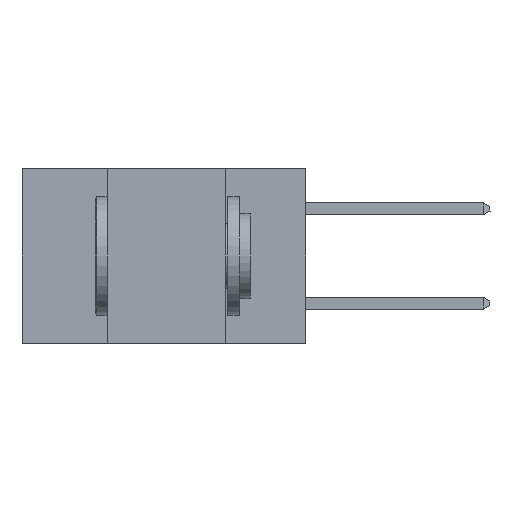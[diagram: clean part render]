
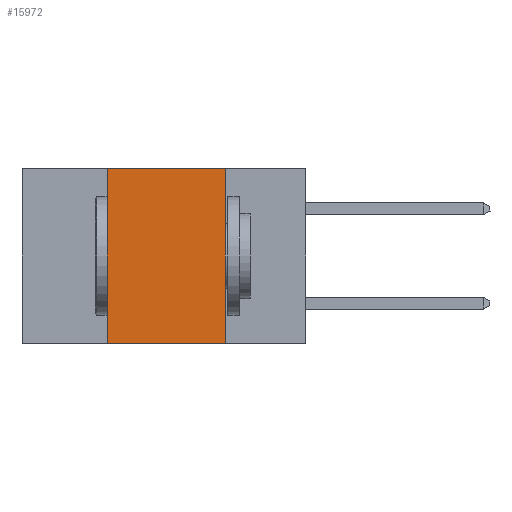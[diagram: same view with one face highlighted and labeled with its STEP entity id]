
A CAD part, left-side view. The second image highlights one B-rep face of the part: STEP entity #15972.
In plain terms, the highlighted planar face has unit normal (-1, 0, 0).
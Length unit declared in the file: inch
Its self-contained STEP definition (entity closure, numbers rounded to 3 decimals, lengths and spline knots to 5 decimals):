
#938 = DIRECTION ( 'NONE',  ( 0., 0., -1. ) ) ;
#1566 = VERTEX_POINT ( 'NONE', #9839 ) ;
#1702 = EDGE_CURVE ( 'NONE', #15841, #10804, #4116, .T. ) ;
#2092 = LINE ( 'NONE', #13589, #2477 ) ;
#2417 = ORIENTED_EDGE ( 'NONE', *, *, #7214, .T. ) ;
#2477 = VECTOR ( 'NONE', #14834, 39.37008 ) ;
#2841 = EDGE_LOOP ( 'NONE', ( #12056, #16413, #3337, #2417 ) ) ;
#3133 = CARTESIAN_POINT ( 'NONE',  ( 0., 0.42, 0. ) ) ;
#3337 = ORIENTED_EDGE ( 'NONE', *, *, #3378, .F. ) ;
#3378 = EDGE_CURVE ( 'NONE', #1566, #9306, #16498, .T. ) ;
#4116 = LINE ( 'NONE', #9894, #16558 ) ;
#4588 = DIRECTION ( 'NONE',  ( 0., -1., 0. ) ) ;
#4719 = CARTESIAN_POINT ( 'NONE',  ( 0., 0.6, 0. ) ) ;
#5078 = CARTESIAN_POINT ( 'NONE',  ( 0., 0.42, 0. ) ) ;
#7214 = EDGE_CURVE ( 'NONE', #1566, #10804, #15994, .T. ) ;
#7483 = DIRECTION ( 'NONE',  ( 0., 0., 1. ) ) ;
#7895 = FACE_OUTER_BOUND ( 'NONE', #2841, .T. ) ;
#8404 = CARTESIAN_POINT ( 'NONE',  ( 0., 0.6, -0.37 ) ) ;
#9306 = VERTEX_POINT ( 'NONE', #3133 ) ;
#9507 = PLANE ( 'NONE',  #12955 ) ;
#9690 = EDGE_CURVE ( 'NONE', #9306, #15841, #2092, .T. ) ;
#9839 = CARTESIAN_POINT ( 'NONE',  ( 0., 0.42, -0.37 ) ) ;
#9894 = CARTESIAN_POINT ( 'NONE',  ( 0., 0.17, 0. ) ) ;
#10804 = VERTEX_POINT ( 'NONE', #12071 ) ;
#11000 = CARTESIAN_POINT ( 'NONE',  ( 0., 0.17, 0. ) ) ;
#12056 = ORIENTED_EDGE ( 'NONE', *, *, #1702, .F. ) ;
#12071 = CARTESIAN_POINT ( 'NONE',  ( 0., 0.17, -0.37 ) ) ;
#12361 = VECTOR ( 'NONE', #4588, 39.37008 ) ;
#12955 = AXIS2_PLACEMENT_3D ( 'NONE', #4719, #13684, #938 ) ;
#13589 = CARTESIAN_POINT ( 'NONE',  ( 0., 0.6, 0. ) ) ;
#13684 = DIRECTION ( 'NONE',  ( 1., 0., 0. ) ) ;
#13706 = DIRECTION ( 'NONE',  ( 0., 0., -1. ) ) ;
#14692 = VECTOR ( 'NONE', #7483, 39.37008 ) ;
#14834 = DIRECTION ( 'NONE',  ( 0., -1., 0. ) ) ;
#15841 = VERTEX_POINT ( 'NONE', #11000 ) ;
#15972 = ADVANCED_FACE ( 'NONE', ( #7895 ), #9507, .F. ) ;
#15994 = LINE ( 'NONE', #8404, #12361 ) ;
#16413 = ORIENTED_EDGE ( 'NONE', *, *, #9690, .F. ) ;
#16498 = LINE ( 'NONE', #5078, #14692 ) ;
#16558 = VECTOR ( 'NONE', #13706, 39.37008 ) ;
